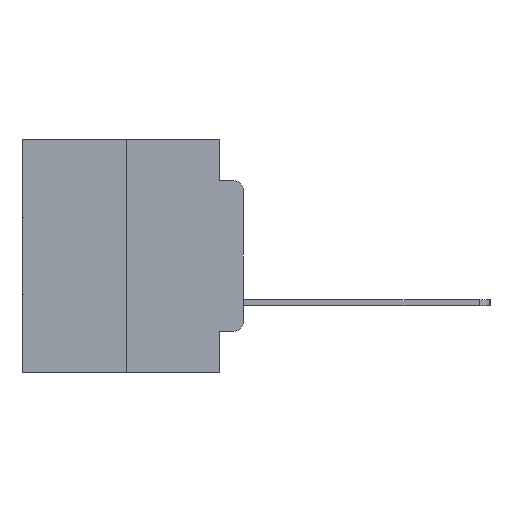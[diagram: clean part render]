
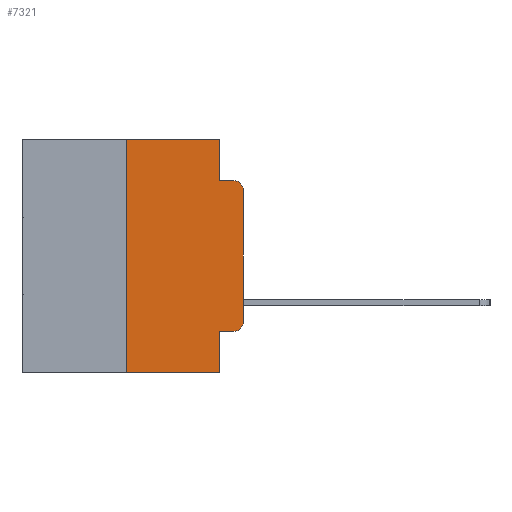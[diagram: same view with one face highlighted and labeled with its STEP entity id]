
A CAD part, left-side view. The second image highlights one B-rep face of the part: STEP entity #7321.
In plain terms, the highlighted planar face has unit normal (-1, 0, 0).
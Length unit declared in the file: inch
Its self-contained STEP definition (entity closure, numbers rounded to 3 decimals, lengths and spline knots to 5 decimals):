
#160 = EDGE_CURVE ( 'NONE', #16937, #13083, #889, .T. ) ;
#487 = ORIENTED_EDGE ( 'NONE', *, *, #10218, .T. ) ;
#861 = CARTESIAN_POINT ( 'NONE',  ( 0., 0.25, -0.5 ) ) ;
#889 = CIRCLE ( 'NONE', #17445, 0.02 ) ;
#1121 = CARTESIAN_POINT ( 'NONE',  ( 0., 0.02, -0.1085 ) ) ;
#1424 = DIRECTION ( 'NONE',  ( -1., 0., 0. ) ) ;
#1788 = EDGE_CURVE ( 'NONE', #10638, #16937, #28125, .T. ) ;
#1813 = DIRECTION ( 'NONE',  ( 0., 0., 1. ) ) ;
#2045 = CARTESIAN_POINT ( 'NONE',  ( 0., 0.473, 0. ) ) ;
#2200 = LINE ( 'NONE', #7698, #13795 ) ;
#2438 = CARTESIAN_POINT ( 'NONE',  ( 0., 0.473, 0. ) ) ;
#3073 = VERTEX_POINT ( 'NONE', #18481 ) ;
#3556 = LINE ( 'NONE', #26801, #26230 ) ;
#4536 = DIRECTION ( 'NONE',  ( 0., 0., -1. ) ) ;
#4828 = DIRECTION ( 'NONE',  ( 1., 0., 0. ) ) ;
#5383 = FACE_OUTER_BOUND ( 'NONE', #24223, .T. ) ;
#5522 = VECTOR ( 'NONE', #1813, 39.37008 ) ;
#5572 = CARTESIAN_POINT ( 'NONE',  ( 0., 0., -0.1085 ) ) ;
#5803 = CARTESIAN_POINT ( 'NONE',  ( 0., 0.051, 0. ) ) ;
#6830 = VERTEX_POINT ( 'NONE', #12455 ) ;
#7321 = ADVANCED_FACE ( 'NONE', ( #5383 ), #16240, .F. ) ;
#7698 = CARTESIAN_POINT ( 'NONE',  ( 0., 0.051, -0.0885 ) ) ;
#8541 = EDGE_CURVE ( 'NONE', #21148, #25659, #13298, .T. ) ;
#9436 = LINE ( 'NONE', #24449, #21432 ) ;
#9929 = VERTEX_POINT ( 'NONE', #14213 ) ;
#10057 = ORIENTED_EDGE ( 'NONE', *, *, #16265, .F. ) ;
#10218 = EDGE_CURVE ( 'NONE', #6830, #10638, #28454, .T. ) ;
#10638 = VERTEX_POINT ( 'NONE', #16904 ) ;
#11216 = DIRECTION ( 'NONE',  ( 0., -1., 0. ) ) ;
#11748 = EDGE_CURVE ( 'NONE', #9929, #6830, #3556, .T. ) ;
#11938 = CARTESIAN_POINT ( 'NONE',  ( 0., 0.02, -0.0885 ) ) ;
#12455 = CARTESIAN_POINT ( 'NONE',  ( 0., 0.02, -0.4115 ) ) ;
#13083 = VERTEX_POINT ( 'NONE', #11938 ) ;
#13255 = ORIENTED_EDGE ( 'NONE', *, *, #1788, .T. ) ;
#13298 = LINE ( 'NONE', #2045, #24488 ) ;
#13317 = DIRECTION ( 'NONE',  ( 0., 0., -1. ) ) ;
#13795 = VECTOR ( 'NONE', #16801, 39.37008 ) ;
#13936 = ORIENTED_EDGE ( 'NONE', *, *, #26680, .F. ) ;
#14004 = DIRECTION ( 'NONE',  ( -1., 0., 0. ) ) ;
#14213 = CARTESIAN_POINT ( 'NONE',  ( 0., 0.051, -0.4115 ) ) ;
#14644 = ORIENTED_EDGE ( 'NONE', *, *, #8541, .F. ) ;
#14756 = EDGE_CURVE ( 'NONE', #9929, #3073, #23346, .T. ) ;
#15282 = CARTESIAN_POINT ( 'NONE',  ( 0., 0.02, -0.3915 ) ) ;
#15841 = AXIS2_PLACEMENT_3D ( 'NONE', #15282, #1424, #17515 ) ;
#16240 = PLANE ( 'NONE',  #21165 ) ;
#16265 = EDGE_CURVE ( 'NONE', #26751, #21148, #17657, .T. ) ;
#16801 = DIRECTION ( 'NONE',  ( 0., -1., 0. ) ) ;
#16904 = CARTESIAN_POINT ( 'NONE',  ( 0., 0., -0.3915 ) ) ;
#16937 = VERTEX_POINT ( 'NONE', #5572 ) ;
#17042 = VECTOR ( 'NONE', #23316, 39.37008 ) ;
#17445 = AXIS2_PLACEMENT_3D ( 'NONE', #1121, #14004, #4536 ) ;
#17515 = DIRECTION ( 'NONE',  ( 0., 0., -1. ) ) ;
#17657 = LINE ( 'NONE', #28884, #5522 ) ;
#18481 = CARTESIAN_POINT ( 'NONE',  ( 0., 0.051, -0.5 ) ) ;
#19206 = VECTOR ( 'NONE', #27719, 39.37008 ) ;
#19431 = DIRECTION ( 'NONE',  ( 0., 0., -1. ) ) ;
#20471 = VERTEX_POINT ( 'NONE', #23392 ) ;
#20773 = DIRECTION ( 'NONE',  ( 0., 0., -1. ) ) ;
#20799 = EDGE_CURVE ( 'NONE', #25659, #20471, #9436, .T. ) ;
#21118 = CARTESIAN_POINT ( 'NONE',  ( 0., 0.473, -0.5 ) ) ;
#21148 = VERTEX_POINT ( 'NONE', #27731 ) ;
#21165 = AXIS2_PLACEMENT_3D ( 'NONE', #2438, #4828, #20773 ) ;
#21432 = VECTOR ( 'NONE', #13317, 39.37008 ) ;
#22023 = ORIENTED_EDGE ( 'NONE', *, *, #22111, .T. ) ;
#22111 = EDGE_CURVE ( 'NONE', #26751, #3073, #25124, .T. ) ;
#23316 = DIRECTION ( 'NONE',  ( 0., 0., 1. ) ) ;
#23346 = LINE ( 'NONE', #5803, #24747 ) ;
#23392 = CARTESIAN_POINT ( 'NONE',  ( 0., 0.051, -0.0885 ) ) ;
#23515 = CARTESIAN_POINT ( 'NONE',  ( 0., 0., 0. ) ) ;
#24102 = ORIENTED_EDGE ( 'NONE', *, *, #11748, .T. ) ;
#24223 = EDGE_LOOP ( 'NONE', ( #13255, #25110, #13936, #25788, #14644, #10057, #22023, #28521, #24102, #487 ) ) ;
#24449 = CARTESIAN_POINT ( 'NONE',  ( 0., 0.051, 0. ) ) ;
#24488 = VECTOR ( 'NONE', #24743, 39.37008 ) ;
#24743 = DIRECTION ( 'NONE',  ( 0., -1., 0. ) ) ;
#24747 = VECTOR ( 'NONE', #19431, 39.37008 ) ;
#25110 = ORIENTED_EDGE ( 'NONE', *, *, #160, .T. ) ;
#25124 = LINE ( 'NONE', #21118, #19206 ) ;
#25659 = VERTEX_POINT ( 'NONE', #28092 ) ;
#25788 = ORIENTED_EDGE ( 'NONE', *, *, #20799, .F. ) ;
#26230 = VECTOR ( 'NONE', #11216, 39.37008 ) ;
#26680 = EDGE_CURVE ( 'NONE', #20471, #13083, #2200, .T. ) ;
#26751 = VERTEX_POINT ( 'NONE', #861 ) ;
#26801 = CARTESIAN_POINT ( 'NONE',  ( 0., 0.051, -0.4115 ) ) ;
#27719 = DIRECTION ( 'NONE',  ( 0., -1., 0. ) ) ;
#27731 = CARTESIAN_POINT ( 'NONE',  ( 0., 0.25, 0. ) ) ;
#28092 = CARTESIAN_POINT ( 'NONE',  ( 0., 0.051, 0. ) ) ;
#28125 = LINE ( 'NONE', #23515, #17042 ) ;
#28454 = CIRCLE ( 'NONE', #15841, 0.02 ) ;
#28521 = ORIENTED_EDGE ( 'NONE', *, *, #14756, .F. ) ;
#28884 = CARTESIAN_POINT ( 'NONE',  ( 0., 0.25, 0. ) ) ;
